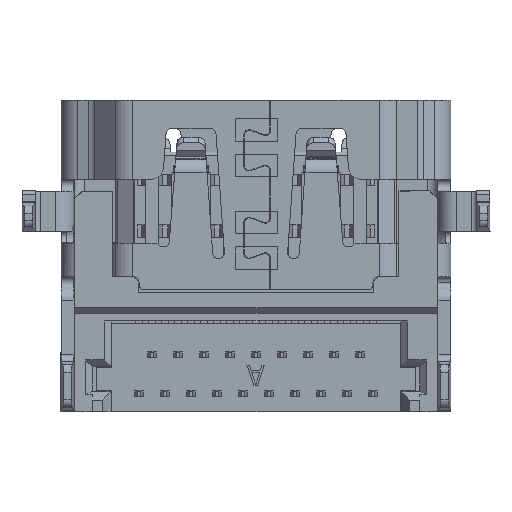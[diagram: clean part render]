
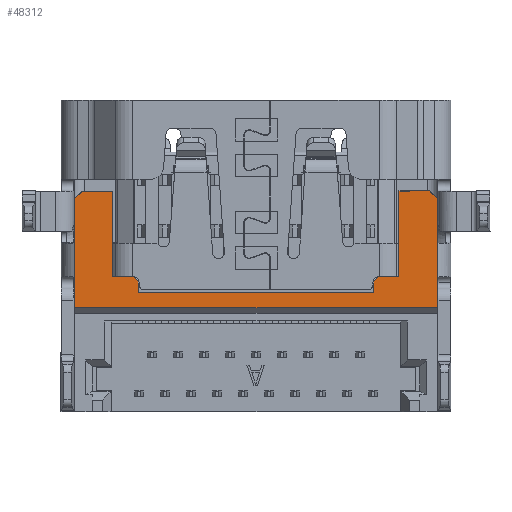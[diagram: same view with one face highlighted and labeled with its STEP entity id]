
A CAD part, front view. The second image highlights one B-rep face of the part: STEP entity #48312.
In plain terms, the highlighted planar face has unit normal (0, -1, 0).
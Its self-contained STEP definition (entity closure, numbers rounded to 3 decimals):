
#123 = CARTESIAN_POINT ( 'NONE',  ( 6.975, -6.01, -3.8 ) ) ;
#883 = VECTOR ( 'NONE', #30647, 1000. ) ;
#2171 = VECTOR ( 'NONE', #9488, 1000. ) ;
#2779 = CARTESIAN_POINT ( 'NONE',  ( -6.975, -6.01, -8. ) ) ;
#3214 = EDGE_CURVE ( 'NONE', #68433, #70473, #39511, .T. ) ;
#3261 = DIRECTION ( 'NONE',  ( 0., 0., -1. ) ) ;
#3605 = VECTOR ( 'NONE', #55792, 1000. ) ;
#3642 = ORIENTED_EDGE ( 'NONE', *, *, #20916, .T. ) ;
#3712 = VERTEX_POINT ( 'NONE', #3870 ) ;
#3870 = CARTESIAN_POINT ( 'NONE',  ( 4.525, -6.01, -7. ) ) ;
#4335 = DIRECTION ( 'NONE',  ( 1., 0., 0. ) ) ;
#4675 = EDGE_CURVE ( 'NONE', #30113, #66026, #62234, .T. ) ;
#5064 = CARTESIAN_POINT ( 'NONE',  ( -4.525, -6.01, -7. ) ) ;
#5319 = DIRECTION ( 'NONE',  ( 0., 0., -1. ) ) ;
#5563 = CARTESIAN_POINT ( 'NONE',  ( 6.975, -6.01, -3.8 ) ) ;
#5652 = ORIENTED_EDGE ( 'NONE', *, *, #58706, .T. ) ;
#6658 = LINE ( 'NONE', #48214, #3605 ) ;
#8182 = DIRECTION ( 'NONE',  ( 0., -1., 0. ) ) ;
#8867 = VERTEX_POINT ( 'NONE', #50917 ) ;
#9488 = DIRECTION ( 'NONE',  ( -1., 0., 0. ) ) ;
#10529 = CARTESIAN_POINT ( 'NONE',  ( -4.725, -6.01, -6.8 ) ) ;
#11455 = CARTESIAN_POINT ( 'NONE',  ( 5.5, -6.01, -3.5 ) ) ;
#11985 = VECTOR ( 'NONE', #57381, 1000. ) ;
#12093 = VECTOR ( 'NONE', #36972, 1000. ) ;
#12120 = CARTESIAN_POINT ( 'NONE',  ( -6.975, -6.01, -3.8 ) ) ;
#12920 = EDGE_CURVE ( 'NONE', #8867, #70473, #6658, .T. ) ;
#13428 = ORIENTED_EDGE ( 'NONE', *, *, #58032, .T. ) ;
#13904 = VECTOR ( 'NONE', #50268, 1000. ) ;
#14450 = CARTESIAN_POINT ( 'NONE',  ( 5.5, -6.01, -3.5 ) ) ;
#15005 = VECTOR ( 'NONE', #64289, 1000. ) ;
#15945 = CARTESIAN_POINT ( 'NONE',  ( -6.975, -6.01, -3.8 ) ) ;
#16068 = ORIENTED_EDGE ( 'NONE', *, *, #66648, .T. ) ;
#16968 = VECTOR ( 'NONE', #30848, 1000. ) ;
#17278 = CARTESIAN_POINT ( 'NONE',  ( -5.5, -6.01, -6.8 ) ) ;
#17298 = LINE ( 'NONE', #58462, #42051 ) ;
#18743 = DIRECTION ( 'NONE',  ( -1., 0., 0. ) ) ;
#19588 = VECTOR ( 'NONE', #70519, 1000. ) ;
#20916 = EDGE_CURVE ( 'NONE', #68433, #66026, #71829, .T. ) ;
#20947 = VECTOR ( 'NONE', #3261, 1000. ) ;
#21970 = EDGE_LOOP ( 'NONE', ( #5652, #55526, #68721, #39596, #25375, #56664, #45980, #3642, #48232, #53054, #32153, #13428, #16068, #64939, #26187, #41592 ) ) ;
#22121 = CARTESIAN_POINT ( 'NONE',  ( 6.675, -6.01, -3.5 ) ) ;
#22684 = CARTESIAN_POINT ( 'NONE',  ( 6.975, -6.01, -3.5 ) ) ;
#22862 = CARTESIAN_POINT ( 'NONE',  ( 4.725, -6.01, -6.8 ) ) ;
#23241 = LINE ( 'NONE', #77937, #73192 ) ;
#23546 = CARTESIAN_POINT ( 'NONE',  ( -5.5, -6.01, -3.5 ) ) ;
#24235 = EDGE_CURVE ( 'NONE', #53717, #72177, #61168, .T. ) ;
#24772 = EDGE_CURVE ( 'NONE', #30113, #54689, #47914, .T. ) ;
#25375 = ORIENTED_EDGE ( 'NONE', *, *, #72741, .T. ) ;
#26180 = CARTESIAN_POINT ( 'NONE',  ( 6.975, -6.01, -3.5 ) ) ;
#26187 = ORIENTED_EDGE ( 'NONE', *, *, #66707, .T. ) ;
#26363 = AXIS2_PLACEMENT_3D ( 'NONE', #26180, #8182, #33365 ) ;
#26580 = FACE_OUTER_BOUND ( 'NONE', #21970, .T. ) ;
#27839 = VERTEX_POINT ( 'NONE', #11455 ) ;
#30113 = VERTEX_POINT ( 'NONE', #123 ) ;
#30234 = CARTESIAN_POINT ( 'NONE',  ( -4.525, -6.01, -3.5 ) ) ;
#30361 = VECTOR ( 'NONE', #71778, 1000. ) ;
#30647 = DIRECTION ( 'NONE',  ( -1., 0., 0. ) ) ;
#30848 = DIRECTION ( 'NONE',  ( 1., 0., 0. ) ) ;
#30866 = VERTEX_POINT ( 'NONE', #71026 ) ;
#32153 = ORIENTED_EDGE ( 'NONE', *, *, #61486, .T. ) ;
#32993 = LINE ( 'NONE', #37794, #11985 ) ;
#33365 = DIRECTION ( 'NONE',  ( 0., 0., -1. ) ) ;
#35819 = LINE ( 'NONE', #5064, #30361 ) ;
#36576 = LINE ( 'NONE', #30234, #12093 ) ;
#36784 = CARTESIAN_POINT ( 'NONE',  ( 4.525, -6.01, -7.4 ) ) ;
#36972 = DIRECTION ( 'NONE',  ( 0., 0., 1. ) ) ;
#37000 = LINE ( 'NONE', #60588, #883 ) ;
#37078 = CARTESIAN_POINT ( 'NONE',  ( 6.975, -6.01, -3.8 ) ) ;
#37794 = CARTESIAN_POINT ( 'NONE',  ( 4.725, -6.01, -6.8 ) ) ;
#38046 = EDGE_CURVE ( 'NONE', #57719, #61843, #55492, .T. ) ;
#38241 = VECTOR ( 'NONE', #46851, 1000. ) ;
#38724 = EDGE_CURVE ( 'NONE', #53003, #3712, #32993, .T. ) ;
#39140 = CARTESIAN_POINT ( 'NONE',  ( 4.525, -6.01, -7.4 ) ) ;
#39511 = LINE ( 'NONE', #15945, #15005 ) ;
#39596 = ORIENTED_EDGE ( 'NONE', *, *, #58034, .T. ) ;
#41183 = DIRECTION ( 'NONE',  ( 0., 0., 1. ) ) ;
#41592 = ORIENTED_EDGE ( 'NONE', *, *, #24235, .F. ) ;
#42051 = VECTOR ( 'NONE', #5319, 1000. ) ;
#45980 = ORIENTED_EDGE ( 'NONE', *, *, #3214, .F. ) ;
#46372 = VECTOR ( 'NONE', #18743, 1000. ) ;
#46851 = DIRECTION ( 'NONE',  ( -1., 0., 0. ) ) ;
#47256 = CARTESIAN_POINT ( 'NONE',  ( 6.975, -6.01, -6.8 ) ) ;
#47914 = LINE ( 'NONE', #5563, #19588 ) ;
#48214 = CARTESIAN_POINT ( 'NONE',  ( -6.675, -6.01, -3.5 ) ) ;
#48232 = ORIENTED_EDGE ( 'NONE', *, *, #4675, .F. ) ;
#48312 = ADVANCED_FACE ( 'NONE', ( #26580 ), #57344, .T. ) ;
#49212 = CARTESIAN_POINT ( 'NONE',  ( 6.975, -6.01, -8. ) ) ;
#50268 = DIRECTION ( 'NONE',  ( 0., 0., -1. ) ) ;
#50917 = CARTESIAN_POINT ( 'NONE',  ( -6.675, -6.01, -3.5 ) ) ;
#51693 = VERTEX_POINT ( 'NONE', #23546 ) ;
#53003 = VERTEX_POINT ( 'NONE', #22862 ) ;
#53054 = ORIENTED_EDGE ( 'NONE', *, *, #24772, .T. ) ;
#53717 = VERTEX_POINT ( 'NONE', #78845 ) ;
#54689 = VERTEX_POINT ( 'NONE', #22121 ) ;
#55492 = LINE ( 'NONE', #66299, #46372 ) ;
#55526 = ORIENTED_EDGE ( 'NONE', *, *, #63852, .T. ) ;
#55792 = DIRECTION ( 'NONE',  ( -0.707, 0., -0.707 ) ) ;
#56088 = VERTEX_POINT ( 'NONE', #66521 ) ;
#56664 = ORIENTED_EDGE ( 'NONE', *, *, #12920, .T. ) ;
#56811 = LINE ( 'NONE', #14450, #20947 ) ;
#57344 = PLANE ( 'NONE',  #26363 ) ;
#57381 = DIRECTION ( 'NONE',  ( -0.707, 0., -0.707 ) ) ;
#57719 = VERTEX_POINT ( 'NONE', #10529 ) ;
#58032 = EDGE_CURVE ( 'NONE', #27839, #30866, #56811, .T. ) ;
#58034 = EDGE_CURVE ( 'NONE', #61843, #51693, #23241, .T. ) ;
#58462 = CARTESIAN_POINT ( 'NONE',  ( 4.525, -6.01, -3.5 ) ) ;
#58706 = EDGE_CURVE ( 'NONE', #53717, #56088, #36576, .T. ) ;
#60588 = CARTESIAN_POINT ( 'NONE',  ( 6.975, -6.01, -3.5 ) ) ;
#61168 = LINE ( 'NONE', #36784, #16968 ) ;
#61486 = EDGE_CURVE ( 'NONE', #54689, #27839, #77381, .T. ) ;
#61843 = VERTEX_POINT ( 'NONE', #17278 ) ;
#62234 = LINE ( 'NONE', #37078, #13904 ) ;
#63852 = EDGE_CURVE ( 'NONE', #56088, #57719, #35819, .T. ) ;
#64289 = DIRECTION ( 'NONE',  ( 0., 0., 1. ) ) ;
#64939 = ORIENTED_EDGE ( 'NONE', *, *, #38724, .T. ) ;
#65841 = CARTESIAN_POINT ( 'NONE',  ( 6.975, -6.01, -8. ) ) ;
#66026 = VERTEX_POINT ( 'NONE', #49212 ) ;
#66299 = CARTESIAN_POINT ( 'NONE',  ( 6.975, -6.01, -6.8 ) ) ;
#66521 = CARTESIAN_POINT ( 'NONE',  ( -4.525, -6.01, -7. ) ) ;
#66648 = EDGE_CURVE ( 'NONE', #30866, #53003, #77213, .T. ) ;
#66707 = EDGE_CURVE ( 'NONE', #3712, #72177, #17298, .T. ) ;
#68433 = VERTEX_POINT ( 'NONE', #2779 ) ;
#68721 = ORIENTED_EDGE ( 'NONE', *, *, #38046, .T. ) ;
#70473 = VERTEX_POINT ( 'NONE', #12120 ) ;
#70519 = DIRECTION ( 'NONE',  ( -0.707, 0., 0.707 ) ) ;
#71026 = CARTESIAN_POINT ( 'NONE',  ( 5.5, -6.01, -6.8 ) ) ;
#71778 = DIRECTION ( 'NONE',  ( -0.707, 0., 0.707 ) ) ;
#71829 = LINE ( 'NONE', #65841, #72886 ) ;
#72177 = VERTEX_POINT ( 'NONE', #39140 ) ;
#72741 = EDGE_CURVE ( 'NONE', #51693, #8867, #37000, .T. ) ;
#72886 = VECTOR ( 'NONE', #4335, 1000. ) ;
#73192 = VECTOR ( 'NONE', #41183, 1000. ) ;
#77213 = LINE ( 'NONE', #47256, #38241 ) ;
#77381 = LINE ( 'NONE', #22684, #2171 ) ;
#77937 = CARTESIAN_POINT ( 'NONE',  ( -5.5, -6.01, -3.5 ) ) ;
#78845 = CARTESIAN_POINT ( 'NONE',  ( -4.525, -6.01, -7.4 ) ) ;
